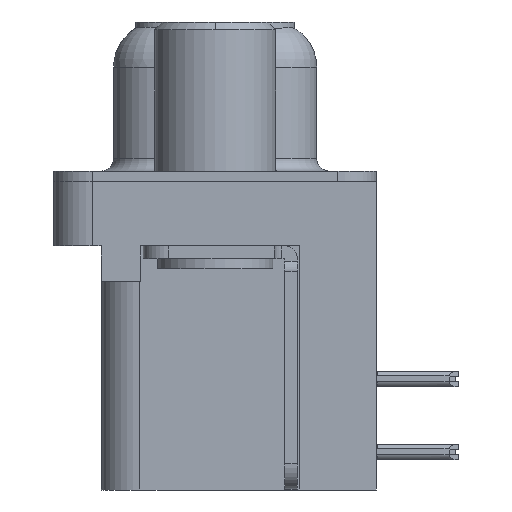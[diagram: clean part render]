
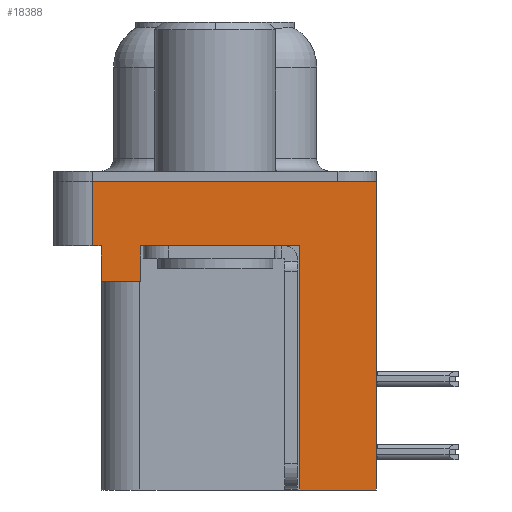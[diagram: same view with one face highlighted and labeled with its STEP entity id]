
A CAD part, left-side view. The second image highlights one B-rep face of the part: STEP entity #18388.
In plain terms, the highlighted planar face has unit normal (-1, 0, 0).
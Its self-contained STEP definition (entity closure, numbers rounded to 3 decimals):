
#42 = ORIENTED_EDGE ( 'NONE', *, *, #1453, .T. ) ;
#1391 = LINE ( 'NONE', #5957, #10984 ) ;
#1453 = EDGE_CURVE ( 'NONE', #5699, #8236, #12021, .T. ) ;
#2484 = VECTOR ( 'NONE', #26403, 1000. ) ;
#2582 = CARTESIAN_POINT ( 'NONE',  ( -2.935, 4.775, -2.5 ) ) ;
#2844 = LINE ( 'NONE', #8806, #15053 ) ;
#3240 = EDGE_CURVE ( 'NONE', #24263, #18671, #26518, .T. ) ;
#3379 = CARTESIAN_POINT ( 'NONE',  ( -2.935, -6.275, -12. ) ) ;
#3496 = DIRECTION ( 'NONE',  ( 0., 1., 0. ) ) ;
#4088 = ORIENTED_EDGE ( 'NONE', *, *, #17008, .F. ) ;
#4453 = CARTESIAN_POINT ( 'NONE',  ( -2.935, 4.425, -2.5 ) ) ;
#4634 = DIRECTION ( 'NONE',  ( 0., 0., 1. ) ) ;
#4645 = VECTOR ( 'NONE', #20054, 1000. ) ;
#5302 = DIRECTION ( 'NONE',  ( 0., -1., 0. ) ) ;
#5456 = CARTESIAN_POINT ( 'NONE',  ( -2.935, 4.425, -3.9 ) ) ;
#5481 = CARTESIAN_POINT ( 'NONE',  ( -2.935, -6.275, 0. ) ) ;
#5553 = CARTESIAN_POINT ( 'NONE',  ( -2.935, 2.895, -3.9 ) ) ;
#5650 = CARTESIAN_POINT ( 'NONE',  ( -2.935, -6.275, -2.5 ) ) ;
#5699 = VERTEX_POINT ( 'NONE', #3379 ) ;
#5957 = CARTESIAN_POINT ( 'NONE',  ( -2.935, 2.895, -3.9 ) ) ;
#6596 = DIRECTION ( 'NONE',  ( 0., 0., 1. ) ) ;
#6661 = EDGE_LOOP ( 'NONE', ( #9508, #4088, #21575, #14780, #17001, #14915, #23931, #12311, #19052, #42 ) ) ;
#6782 = EDGE_CURVE ( 'NONE', #14684, #11237, #23409, .T. ) ;
#6915 = CARTESIAN_POINT ( 'NONE',  ( -2.935, 2.895, -2.5 ) ) ;
#7613 = VECTOR ( 'NONE', #5302, 1000. ) ;
#8236 = VERTEX_POINT ( 'NONE', #19882 ) ;
#8582 = CARTESIAN_POINT ( 'NONE',  ( -2.935, 4.775, -2.5 ) ) ;
#8806 = CARTESIAN_POINT ( 'NONE',  ( -2.935, 4.425, -3.9 ) ) ;
#9508 = ORIENTED_EDGE ( 'NONE', *, *, #15258, .F. ) ;
#9858 = EDGE_CURVE ( 'NONE', #14684, #10029, #1391, .T. ) ;
#10029 = VERTEX_POINT ( 'NONE', #6915 ) ;
#10811 = VECTOR ( 'NONE', #3496, 1000. ) ;
#10984 = VECTOR ( 'NONE', #12203, 1000. ) ;
#11136 = DIRECTION ( 'NONE',  ( 0., -1., 0. ) ) ;
#11237 = VERTEX_POINT ( 'NONE', #20652 ) ;
#12011 = CARTESIAN_POINT ( 'NONE',  ( -2.935, -3.295, -12. ) ) ;
#12021 = LINE ( 'NONE', #5650, #4645 ) ;
#12058 = LINE ( 'NONE', #14295, #13670 ) ;
#12203 = DIRECTION ( 'NONE',  ( 0., 0., 1. ) ) ;
#12311 = ORIENTED_EDGE ( 'NONE', *, *, #25663, .F. ) ;
#12383 = DIRECTION ( 'NONE',  ( 0., 1., 0. ) ) ;
#12754 = LINE ( 'NONE', #12011, #2484 ) ;
#13270 = CARTESIAN_POINT ( 'NONE',  ( -2.935, -6.275, -2.5 ) ) ;
#13524 = CARTESIAN_POINT ( 'NONE',  ( -2.935, -6.275, -2.5 ) ) ;
#13670 = VECTOR ( 'NONE', #12383, 1000. ) ;
#13721 = LINE ( 'NONE', #5481, #7613 ) ;
#13981 = VECTOR ( 'NONE', #4634, 1000. ) ;
#14295 = CARTESIAN_POINT ( 'NONE',  ( -2.935, -3.295, -12. ) ) ;
#14350 = CARTESIAN_POINT ( 'NONE',  ( -2.935, -3.295, -2.5 ) ) ;
#14568 = VERTEX_POINT ( 'NONE', #26327 ) ;
#14684 = VERTEX_POINT ( 'NONE', #5553 ) ;
#14780 = ORIENTED_EDGE ( 'NONE', *, *, #23084, .F. ) ;
#14915 = ORIENTED_EDGE ( 'NONE', *, *, #9858, .T. ) ;
#15053 = VECTOR ( 'NONE', #6596, 1000. ) ;
#15258 = EDGE_CURVE ( 'NONE', #17120, #8236, #13721, .T. ) ;
#16461 = EDGE_CURVE ( 'NONE', #5699, #14568, #12058, .T. ) ;
#17001 = ORIENTED_EDGE ( 'NONE', *, *, #6782, .F. ) ;
#17008 = EDGE_CURVE ( 'NONE', #24263, #17120, #21101, .T. ) ;
#17120 = VERTEX_POINT ( 'NONE', #25313 ) ;
#17140 = VECTOR ( 'NONE', #19743, 1000. ) ;
#18388 = ADVANCED_FACE ( 'NONE', ( #24266 ), #24203, .T. ) ;
#18427 = EDGE_CURVE ( 'NONE', #10029, #26219, #18747, .T. ) ;
#18671 = VERTEX_POINT ( 'NONE', #4453 ) ;
#18747 = LINE ( 'NONE', #13524, #17140 ) ;
#19052 = ORIENTED_EDGE ( 'NONE', *, *, #16461, .F. ) ;
#19743 = DIRECTION ( 'NONE',  ( 0., -1., 0. ) ) ;
#19882 = CARTESIAN_POINT ( 'NONE',  ( -2.935, -6.275, 0. ) ) ;
#20054 = DIRECTION ( 'NONE',  ( 0., 0., 1. ) ) ;
#20652 = CARTESIAN_POINT ( 'NONE',  ( -2.935, 4.425, -3.9 ) ) ;
#21101 = LINE ( 'NONE', #2582, #13981 ) ;
#21575 = ORIENTED_EDGE ( 'NONE', *, *, #3240, .T. ) ;
#21719 = AXIS2_PLACEMENT_3D ( 'NONE', #26287, #24021, #26115 ) ;
#23084 = EDGE_CURVE ( 'NONE', #11237, #18671, #2844, .T. ) ;
#23409 = LINE ( 'NONE', #5456, #10811 ) ;
#23931 = ORIENTED_EDGE ( 'NONE', *, *, #18427, .T. ) ;
#24021 = DIRECTION ( 'NONE',  ( -1., 0., 0. ) ) ;
#24203 = PLANE ( 'NONE',  #21719 ) ;
#24263 = VERTEX_POINT ( 'NONE', #8582 ) ;
#24266 = FACE_OUTER_BOUND ( 'NONE', #6661, .T. ) ;
#24573 = VECTOR ( 'NONE', #11136, 1000. ) ;
#25313 = CARTESIAN_POINT ( 'NONE',  ( -2.935, 4.775, 0. ) ) ;
#25663 = EDGE_CURVE ( 'NONE', #14568, #26219, #12754, .T. ) ;
#26115 = DIRECTION ( 'NONE',  ( 0., 0., 1. ) ) ;
#26219 = VERTEX_POINT ( 'NONE', #14350 ) ;
#26287 = CARTESIAN_POINT ( 'NONE',  ( -2.935, -6.275, -2.5 ) ) ;
#26327 = CARTESIAN_POINT ( 'NONE',  ( -2.935, -3.295, -12. ) ) ;
#26403 = DIRECTION ( 'NONE',  ( 0., 0., 1. ) ) ;
#26518 = LINE ( 'NONE', #13270, #24573 ) ;
